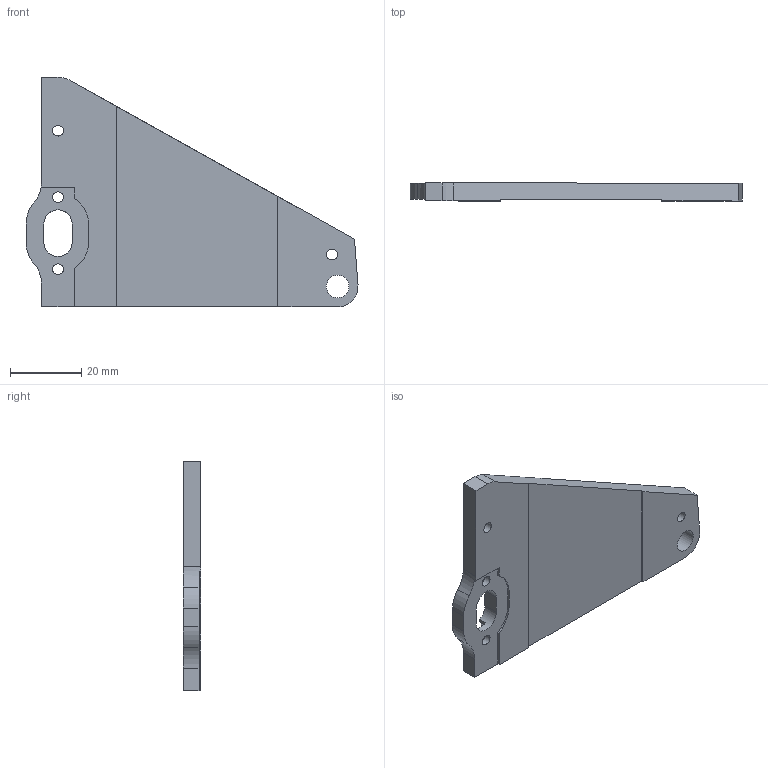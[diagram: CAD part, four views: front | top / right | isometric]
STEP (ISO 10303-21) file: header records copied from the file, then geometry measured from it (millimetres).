
FILE_DESCRIPTION (( 'STEP AP214' ), '1' );
FILE_NAME ('JT_Mag_Well_Right.step', '2016-01-30T20:06:08', ( 'WarFairy' ), ( '' ), 'SwSTEP 2.0', 'SolidWorks 2015', '' );
FILE_SCHEMA (( 'AUTOMOTIVE_DESIGN' ));
Length unit declared in the file: millimetre
Products named in the file (1): JT_Mag_Well_Right
Bounding box: 93 x 5 x 64.36 mm (x, y, z)
Volume: 17257.2 mm3; surface area: 9326.4 mm2
Topology: 1 solids, 1 shells, 65 faces, 185 edges, 124 vertices
Faces by surface type: plane 50, cylinder 15
Full cylindrical faces by diameter (mm): 3 x4, 6.35 x1
Entity records: 2125 total; most frequent: CARTESIAN_POINT 366, ORIENTED_EDGE 356, DIRECTION 345, EDGE_CURVE 178, VECTOR 143, LINE 143, VERTEX_POINT 122, AXIS2_PLACEMENT_3D 101
